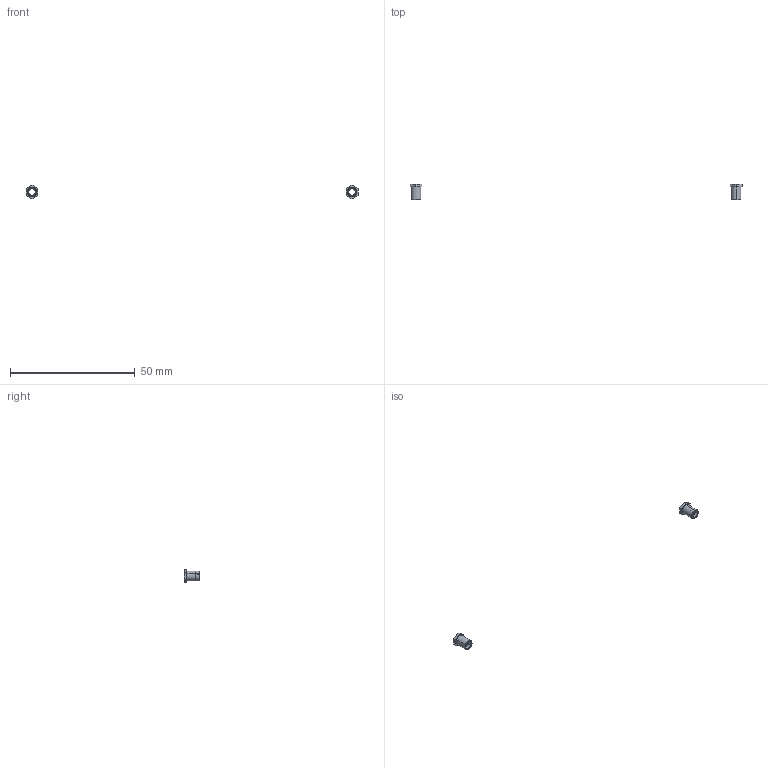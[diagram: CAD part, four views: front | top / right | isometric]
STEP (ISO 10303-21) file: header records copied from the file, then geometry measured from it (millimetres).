
FILE_DESCRIPTION (( 'STEP AP203' ), '1' );
FILE_NAME ('346-072-560-207.STEP', '2022-05-25T01:12:35', ( '' ), ( '' ), 'SwSTEP 2.0', 'SolidWorks 2020', '' );
FILE_SCHEMA (( 'CONFIG_CONTROL_DESIGN' ));
Length unit declared in the file: inch
Products named in the file (4): 345-292-001_560 Tail; 346-072-560-207; 346 Part_Flush Mounting Lugs - 0.156 Dia-TI; 345-250-001_345-250-005-103
Assembly tree (75 placements, depth 2):
  346-072-560-207
    346 Part_Flush Mounting Lugs - 0.156 Dia-TI
    345-292-001_560 Tail  x72
    345-250-001_345-250-005-103  x2
Bounding box: 132.89 x 6.1 x 5.48 mm (x, y, z)
Volume: 92.4 mm3; surface area: 312.9 mm2
Topology: 2 solids, 2 shells, 46 faces, 100 edges, 60 vertices
Faces by surface type: plane 18, cone 12, cylinder 12, torus 4
Entity records: 25576 total; most frequent: CARTESIAN_POINT 4207, ORIENTED_EDGE 4134, DIRECTION 3789, EDGE_CURVE 2067, VECTOR 1767, LINE 1767, VERTEX_POINT 1372, AXIS2_PLACEMENT_3D 1011
